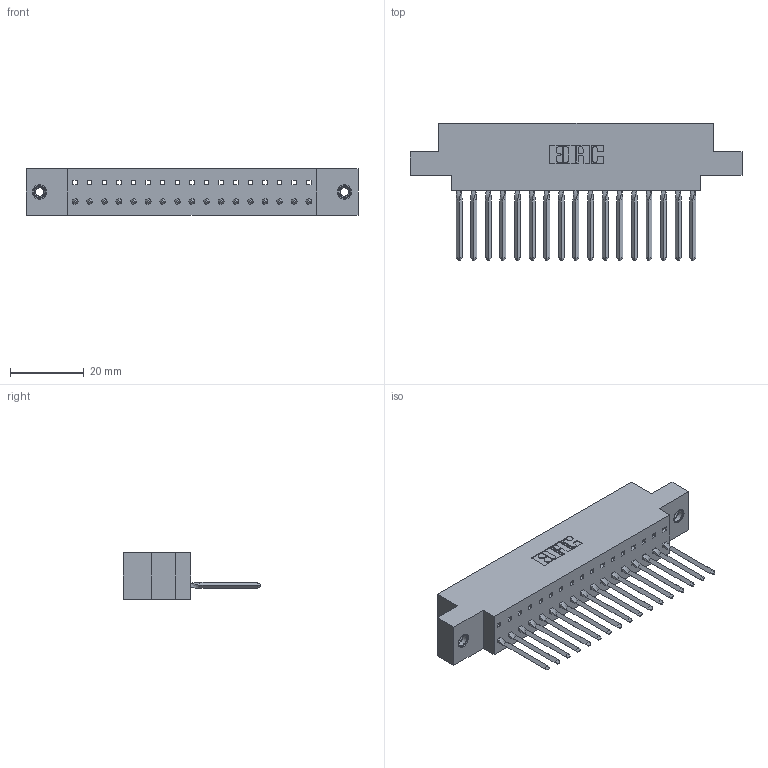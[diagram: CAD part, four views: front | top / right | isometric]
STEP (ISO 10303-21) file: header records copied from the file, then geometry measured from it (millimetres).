
FILE_DESCRIPTION (( 'STEP AP203' ), '1' );
FILE_NAME ('317-017-542-608.STEP', '2020-02-27T15:39:28', ( '' ), ( '' ), 'SwSTEP 2.0', 'SolidWorks 2016', '' );
FILE_SCHEMA (( 'CONFIG_CONTROL_DESIGN' ));
Length unit declared in the file: inch
Products named in the file (4): 345-250-001_345-250-003-102; 317 Part_.156 Dia - TI; 317-017-542-608; 317-290-003_542
Assembly tree (20 placements, depth 2):
  317-017-542-608
    317 Part_.156 Dia - TI
    317-290-003_542  x17
    345-250-001_345-250-003-102  x2
Bounding box: 90.07 x 37.34 x 12.7 mm (x, y, z)
Volume: 13241.9 mm3; surface area: 15616.5 mm2
Topology: 20 solids, 20 shells, 1437 faces, 4100 edges, 2646 vertices
Faces by surface type: plane 1178, cylinder 175, bspline 68, cone 12, torus 4
Entity records: 27720 total; most frequent: CARTESIAN_POINT 5131, ORIENTED_EDGE 4804, DIRECTION 4090, EDGE_CURVE 2402, VECTOR 2212, LINE 2212, VERTEX_POINT 1592, AXIS2_PLACEMENT_3D 939
